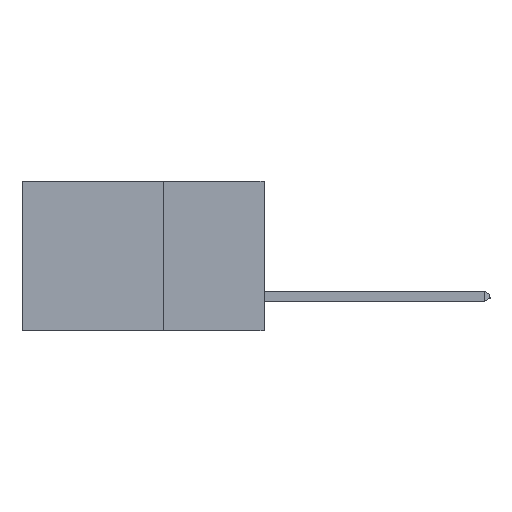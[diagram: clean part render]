
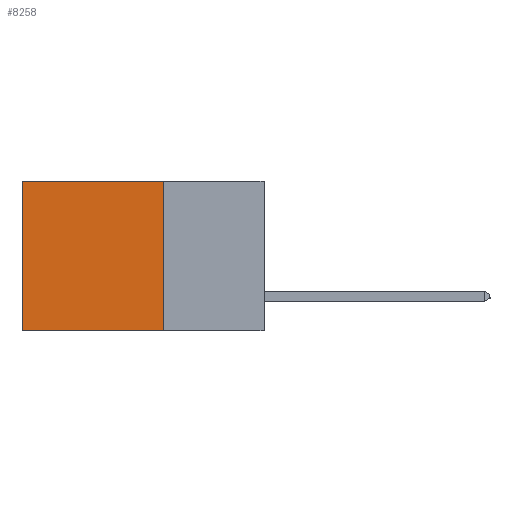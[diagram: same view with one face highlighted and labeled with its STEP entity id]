
A CAD part, left-side view. The second image highlights one B-rep face of the part: STEP entity #8258.
In plain terms, the highlighted planar face has unit normal (-1, 0, 0).
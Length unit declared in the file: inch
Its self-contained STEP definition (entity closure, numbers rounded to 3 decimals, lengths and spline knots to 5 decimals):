
#423 = DIRECTION ( 'NONE',  ( 0., 1., 0. ) ) ;
#882 = ORIENTED_EDGE ( 'NONE', *, *, #13398, .T. ) ;
#1788 = CARTESIAN_POINT ( 'NONE',  ( 0.298, 0.25, 0. ) ) ;
#2359 = VECTOR ( 'NONE', #11916, 39.37008 ) ;
#2774 = LINE ( 'NONE', #10597, #2359 ) ;
#3159 = CARTESIAN_POINT ( 'NONE',  ( 0.298, 0.25, 0. ) ) ;
#3621 = CARTESIAN_POINT ( 'NONE',  ( 0.298, 0.6, 0. ) ) ;
#3816 = VECTOR ( 'NONE', #13355, 39.37008 ) ;
#4545 = PLANE ( 'NONE',  #4616 ) ;
#4571 = ORIENTED_EDGE ( 'NONE', *, *, #10638, .F. ) ;
#4616 = AXIS2_PLACEMENT_3D ( 'NONE', #3159, #13819, #5934 ) ;
#5692 = VECTOR ( 'NONE', #423, 39.37008 ) ;
#5934 = DIRECTION ( 'NONE',  ( 0., 0., -1. ) ) ;
#6115 = VERTEX_POINT ( 'NONE', #6458 ) ;
#6294 = VERTEX_POINT ( 'NONE', #11622 ) ;
#6458 = CARTESIAN_POINT ( 'NONE',  ( 0.298, 0.25, -0.37 ) ) ;
#6601 = FACE_OUTER_BOUND ( 'NONE', #7341, .T. ) ;
#7341 = EDGE_LOOP ( 'NONE', ( #882, #4571, #11220, #8812 ) ) ;
#7940 = LINE ( 'NONE', #12116, #3816 ) ;
#8258 = ADVANCED_FACE ( 'NONE', ( #6601 ), #4545, .F. ) ;
#8668 = DIRECTION ( 'NONE',  ( 0., 0., -1. ) ) ;
#8812 = ORIENTED_EDGE ( 'NONE', *, *, #13522, .T. ) ;
#10597 = CARTESIAN_POINT ( 'NONE',  ( 0.298, 0.6, 0. ) ) ;
#10638 = EDGE_CURVE ( 'NONE', #6115, #6294, #16108, .T. ) ;
#10909 = VERTEX_POINT ( 'NONE', #3621 ) ;
#11220 = ORIENTED_EDGE ( 'NONE', *, *, #11965, .F. ) ;
#11622 = CARTESIAN_POINT ( 'NONE',  ( 0.298, 0.6, -0.37 ) ) ;
#11916 = DIRECTION ( 'NONE',  ( 0., 0., -1. ) ) ;
#11965 = EDGE_CURVE ( 'NONE', #16338, #6115, #17046, .T. ) ;
#12116 = CARTESIAN_POINT ( 'NONE',  ( 0.298, 0.25, 0. ) ) ;
#12961 = CARTESIAN_POINT ( 'NONE',  ( 0.298, 0.25, 0. ) ) ;
#13355 = DIRECTION ( 'NONE',  ( 0., 1., 0. ) ) ;
#13398 = EDGE_CURVE ( 'NONE', #10909, #6294, #2774, .T. ) ;
#13522 = EDGE_CURVE ( 'NONE', #16338, #10909, #7940, .T. ) ;
#13819 = DIRECTION ( 'NONE',  ( 1., 0., 0. ) ) ;
#16108 = LINE ( 'NONE', #16266, #5692 ) ;
#16266 = CARTESIAN_POINT ( 'NONE',  ( 0.298, 0.25, -0.37 ) ) ;
#16338 = VERTEX_POINT ( 'NONE', #12961 ) ;
#16646 = VECTOR ( 'NONE', #8668, 39.37008 ) ;
#17046 = LINE ( 'NONE', #1788, #16646 ) ;
